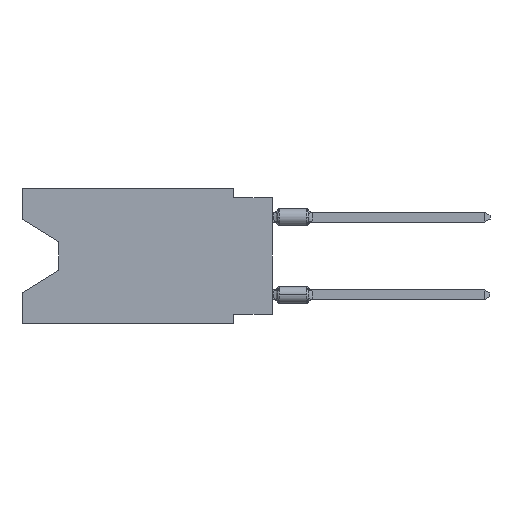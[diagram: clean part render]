
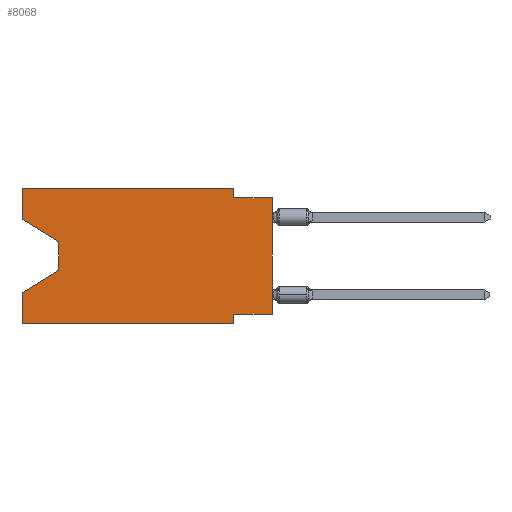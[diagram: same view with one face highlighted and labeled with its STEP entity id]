
A CAD part, left-side view. The second image highlights one B-rep face of the part: STEP entity #8068.
In plain terms, the highlighted planar face has unit normal (-1, 0, 0).
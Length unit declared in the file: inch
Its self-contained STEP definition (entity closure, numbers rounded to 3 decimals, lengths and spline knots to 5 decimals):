
#34 = VERTEX_POINT ( 'NONE', #8624 ) ;
#66 = CARTESIAN_POINT ( 'NONE',  ( 0., 0., -0.025 ) ) ;
#129 = EDGE_CURVE ( 'NONE', #7457, #725, #19513, .T. ) ;
#614 = FACE_OUTER_BOUND ( 'NONE', #7266, .T. ) ;
#715 = ORIENTED_EDGE ( 'NONE', *, *, #19787, .F. ) ;
#725 = VERTEX_POINT ( 'NONE', #18617 ) ;
#905 = CARTESIAN_POINT ( 'NONE',  ( 0., 0.55, -0.138 ) ) ;
#1640 = LINE ( 'NONE', #19847, #15339 ) ;
#1710 = VERTEX_POINT ( 'NONE', #7601 ) ;
#2063 = LINE ( 'NONE', #13725, #12072 ) ;
#2250 = DIRECTION ( 'NONE',  ( 1., 0., 0. ) ) ;
#2414 = LINE ( 'NONE', #12242, #16759 ) ;
#3191 = AXIS2_PLACEMENT_3D ( 'NONE', #10874, #2250, #20879 ) ;
#3193 = VECTOR ( 'NONE', #5909, 39.37008 ) ;
#3466 = VECTOR ( 'NONE', #14336, 39.37008 ) ;
#3709 = CARTESIAN_POINT ( 'NONE',  ( 0., 0.1, -0.35 ) ) ;
#3714 = EDGE_CURVE ( 'NONE', #14697, #10109, #5234, .T. ) ;
#3750 = CARTESIAN_POINT ( 'NONE',  ( 0., 0.645, -0.08025 ) ) ;
#4173 = CARTESIAN_POINT ( 'NONE',  ( 0., 0.645, -0.35 ) ) ;
#4445 = ORIENTED_EDGE ( 'NONE', *, *, #11304, .T. ) ;
#4708 = EDGE_CURVE ( 'NONE', #725, #34, #6707, .T. ) ;
#4816 = DIRECTION ( 'NONE',  ( 0., 0., -1. ) ) ;
#4928 = DIRECTION ( 'NONE',  ( 0., 1., 0. ) ) ;
#5043 = ORIENTED_EDGE ( 'NONE', *, *, #4708, .T. ) ;
#5234 = LINE ( 'NONE', #3709, #14102 ) ;
#5433 = ORIENTED_EDGE ( 'NONE', *, *, #7720, .F. ) ;
#5775 = EDGE_CURVE ( 'NONE', #19356, #10109, #15820, .T. ) ;
#5909 = DIRECTION ( 'NONE',  ( 0., -1., 0. ) ) ;
#6553 = CARTESIAN_POINT ( 'NONE',  ( 0., 0.1, 0. ) ) ;
#6596 = CARTESIAN_POINT ( 'NONE',  ( 0., 0., -0.325 ) ) ;
#6707 = LINE ( 'NONE', #11823, #17968 ) ;
#6772 = EDGE_CURVE ( 'NONE', #1710, #12124, #12389, .T. ) ;
#7059 = ORIENTED_EDGE ( 'NONE', *, *, #13755, .F. ) ;
#7166 = VERTEX_POINT ( 'NONE', #18171 ) ;
#7266 = EDGE_LOOP ( 'NONE', ( #4445, #11115, #5043, #715, #13291, #14813, #15679, #13042, #18133, #9811, #5433, #7059 ) ) ;
#7457 = VERTEX_POINT ( 'NONE', #905 ) ;
#7601 = CARTESIAN_POINT ( 'NONE',  ( 0., 0.1, -0.025 ) ) ;
#7720 = EDGE_CURVE ( 'NONE', #7166, #21355, #2414, .T. ) ;
#7787 = LINE ( 'NONE', #19449, #16669 ) ;
#8039 = VECTOR ( 'NONE', #4816, 39.37008 ) ;
#8068 = ADVANCED_FACE ( 'NONE', ( #614 ), #10766, .F. ) ;
#8514 = LINE ( 'NONE', #6553, #8039 ) ;
#8606 = DIRECTION ( 'NONE',  ( 0., 0., -1. ) ) ;
#8624 = CARTESIAN_POINT ( 'NONE',  ( 0., 0.645, -0.26975 ) ) ;
#8713 = CARTESIAN_POINT ( 'NONE',  ( 0., 0.1, 0. ) ) ;
#9065 = DIRECTION ( 'NONE',  ( 0., -1., 0. ) ) ;
#9796 = VECTOR ( 'NONE', #19197, 39.37008 ) ;
#9811 = ORIENTED_EDGE ( 'NONE', *, *, #18052, .F. ) ;
#10109 = VERTEX_POINT ( 'NONE', #16168 ) ;
#10766 = PLANE ( 'NONE',  #3191 ) ;
#10874 = CARTESIAN_POINT ( 'NONE',  ( 0., 0.645, 0. ) ) ;
#11115 = ORIENTED_EDGE ( 'NONE', *, *, #129, .T. ) ;
#11304 = EDGE_CURVE ( 'NONE', #15997, #7457, #7787, .T. ) ;
#11490 = DIRECTION ( 'NONE',  ( 0., -0.855, -0.519 ) ) ;
#11823 = CARTESIAN_POINT ( 'NONE',  ( 0., 0.55, -0.212 ) ) ;
#12072 = VECTOR ( 'NONE', #17220, 39.37008 ) ;
#12124 = VERTEX_POINT ( 'NONE', #66 ) ;
#12242 = CARTESIAN_POINT ( 'NONE',  ( 0., 0.645, 0. ) ) ;
#12389 = LINE ( 'NONE', #15330, #13999 ) ;
#12909 = LINE ( 'NONE', #17709, #3466 ) ;
#12933 = DIRECTION ( 'NONE',  ( 0., 0., 1. ) ) ;
#13042 = ORIENTED_EDGE ( 'NONE', *, *, #15663, .T. ) ;
#13291 = ORIENTED_EDGE ( 'NONE', *, *, #5775, .T. ) ;
#13447 = DIRECTION ( 'NONE',  ( 0., 0.855, -0.519 ) ) ;
#13725 = CARTESIAN_POINT ( 'NONE',  ( 0., 0.645, 0. ) ) ;
#13755 = EDGE_CURVE ( 'NONE', #15997, #7166, #17621, .T. ) ;
#13978 = CARTESIAN_POINT ( 'NONE',  ( 0., 0.1, -0.325 ) ) ;
#13999 = VECTOR ( 'NONE', #18834, 39.37008 ) ;
#14102 = VECTOR ( 'NONE', #8606, 39.37008 ) ;
#14336 = DIRECTION ( 'NONE',  ( 0., 0., 1. ) ) ;
#14697 = VERTEX_POINT ( 'NONE', #13978 ) ;
#14813 = ORIENTED_EDGE ( 'NONE', *, *, #3714, .F. ) ;
#15330 = CARTESIAN_POINT ( 'NONE',  ( 0., 0., -0.025 ) ) ;
#15339 = VECTOR ( 'NONE', #4928, 39.37008 ) ;
#15663 = EDGE_CURVE ( 'NONE', #20875, #12124, #12909, .T. ) ;
#15679 = ORIENTED_EDGE ( 'NONE', *, *, #18064, .F. ) ;
#15820 = LINE ( 'NONE', #20819, #3193 ) ;
#15997 = VERTEX_POINT ( 'NONE', #3750 ) ;
#16168 = CARTESIAN_POINT ( 'NONE',  ( 0., 0.1, -0.35 ) ) ;
#16669 = VECTOR ( 'NONE', #11490, 39.37008 ) ;
#16759 = VECTOR ( 'NONE', #9065, 39.37008 ) ;
#17220 = DIRECTION ( 'NONE',  ( 0., 0., 1. ) ) ;
#17621 = LINE ( 'NONE', #19362, #21325 ) ;
#17709 = CARTESIAN_POINT ( 'NONE',  ( 0., 0., 0. ) ) ;
#17968 = VECTOR ( 'NONE', #13447, 39.37008 ) ;
#18052 = EDGE_CURVE ( 'NONE', #21355, #1710, #8514, .T. ) ;
#18064 = EDGE_CURVE ( 'NONE', #20875, #14697, #1640, .T. ) ;
#18133 = ORIENTED_EDGE ( 'NONE', *, *, #6772, .F. ) ;
#18171 = CARTESIAN_POINT ( 'NONE',  ( 0., 0.645, 0. ) ) ;
#18617 = CARTESIAN_POINT ( 'NONE',  ( 0., 0.55, -0.212 ) ) ;
#18834 = DIRECTION ( 'NONE',  ( 0., -1., 0. ) ) ;
#19197 = DIRECTION ( 'NONE',  ( 0., 0., -1. ) ) ;
#19356 = VERTEX_POINT ( 'NONE', #4173 ) ;
#19362 = CARTESIAN_POINT ( 'NONE',  ( 0., 0.645, 0. ) ) ;
#19449 = CARTESIAN_POINT ( 'NONE',  ( 0., 0.645, -0.08025 ) ) ;
#19513 = LINE ( 'NONE', #21126, #9796 ) ;
#19787 = EDGE_CURVE ( 'NONE', #19356, #34, #2063, .T. ) ;
#19847 = CARTESIAN_POINT ( 'NONE',  ( 0., 0., -0.325 ) ) ;
#20819 = CARTESIAN_POINT ( 'NONE',  ( 0., 0.645, -0.35 ) ) ;
#20875 = VERTEX_POINT ( 'NONE', #6596 ) ;
#20879 = DIRECTION ( 'NONE',  ( 0., 0., -1. ) ) ;
#21126 = CARTESIAN_POINT ( 'NONE',  ( 0., 0.55, -0.138 ) ) ;
#21325 = VECTOR ( 'NONE', #12933, 39.37008 ) ;
#21355 = VERTEX_POINT ( 'NONE', #8713 ) ;
